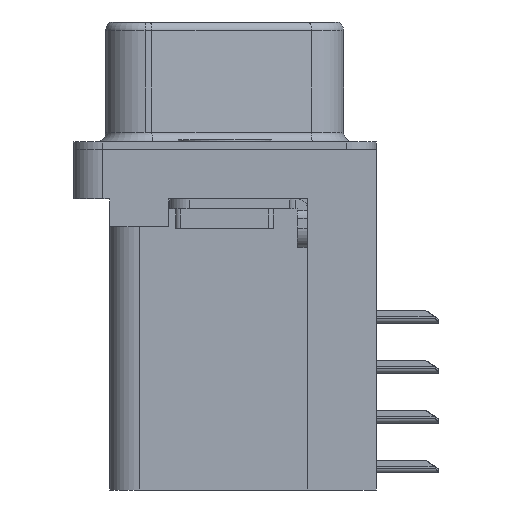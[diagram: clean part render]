
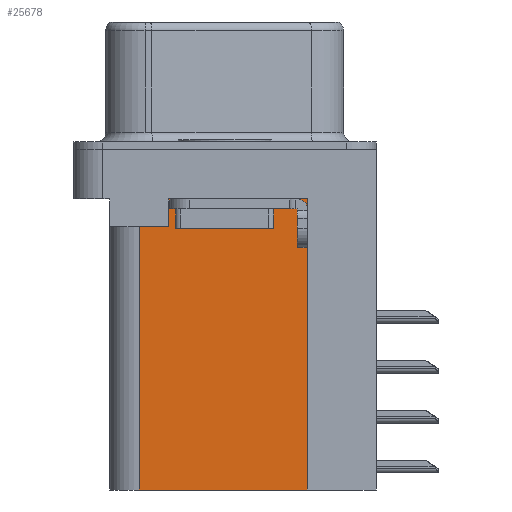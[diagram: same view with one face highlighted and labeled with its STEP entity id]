
A CAD part, left-side view. The second image highlights one B-rep face of the part: STEP entity #25678.
In plain terms, the highlighted planar face has unit normal (-1, 0, 0).
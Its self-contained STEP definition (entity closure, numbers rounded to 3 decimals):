
#505 = EDGE_CURVE ( 'NONE', #12162, #2214, #28429, .T. ) ;
#536 = ORIENTED_EDGE ( 'NONE', *, *, #505, .F. ) ;
#2214 = VERTEX_POINT ( 'NONE', #15525 ) ;
#2223 = ORIENTED_EDGE ( 'NONE', *, *, #35349, .T. ) ;
#3268 = LINE ( 'NONE', #4324, #18031 ) ;
#3417 = CARTESIAN_POINT ( 'NONE',  ( 3.75, 2.85, -3.9 ) ) ;
#3511 = EDGE_CURVE ( 'NONE', #12162, #10727, #16352, .T. ) ;
#3891 = VECTOR ( 'NONE', #4396, 1000. ) ;
#4324 = CARTESIAN_POINT ( 'NONE',  ( 3.75, 4.35, -17.3 ) ) ;
#4396 = DIRECTION ( 'NONE',  ( 0., 1., 0. ) ) ;
#5927 = LINE ( 'NONE', #22564, #13668 ) ;
#7826 = DIRECTION ( 'NONE',  ( 0., 1., 0. ) ) ;
#8161 = VERTEX_POINT ( 'NONE', #13771 ) ;
#8229 = VECTOR ( 'NONE', #20937, 1000. ) ;
#9445 = AXIS2_PLACEMENT_3D ( 'NONE', #10830, #38071, #19734 ) ;
#10727 = VERTEX_POINT ( 'NONE', #12893 ) ;
#10830 = CARTESIAN_POINT ( 'NONE',  ( 3.75, -4.2, -17.3 ) ) ;
#11725 = LINE ( 'NONE', #16073, #3891 ) ;
#12074 = CARTESIAN_POINT ( 'NONE',  ( 3.75, -4.2, -17.3 ) ) ;
#12162 = VERTEX_POINT ( 'NONE', #12074 ) ;
#12893 = CARTESIAN_POINT ( 'NONE',  ( 3.75, -4.2, -2.5 ) ) ;
#13668 = VECTOR ( 'NONE', #7826, 1000. ) ;
#13771 = CARTESIAN_POINT ( 'NONE',  ( 3.75, 2.85, -2.5 ) ) ;
#14056 = EDGE_CURVE ( 'NONE', #23546, #19705, #5927, .T. ) ;
#15314 = ORIENTED_EDGE ( 'NONE', *, *, #3511, .T. ) ;
#15402 = VECTOR ( 'NONE', #32599, 1000. ) ;
#15525 = CARTESIAN_POINT ( 'NONE',  ( 3.75, 4.35, -17.3 ) ) ;
#16073 = CARTESIAN_POINT ( 'NONE',  ( 3.75, -4.2, -2.5 ) ) ;
#16142 = DIRECTION ( 'NONE',  ( 0., 0., 1. ) ) ;
#16352 = LINE ( 'NONE', #33920, #15402 ) ;
#18031 = VECTOR ( 'NONE', #16142, 1000. ) ;
#19467 = EDGE_CURVE ( 'NONE', #10727, #8161, #11725, .T. ) ;
#19604 = PLANE ( 'NONE',  #9445 ) ;
#19705 = VERTEX_POINT ( 'NONE', #20159 ) ;
#19734 = DIRECTION ( 'NONE',  ( 0., 1., 0. ) ) ;
#20159 = CARTESIAN_POINT ( 'NONE',  ( 3.75, 4.35, -3.9 ) ) ;
#20937 = DIRECTION ( 'NONE',  ( 0., 0., -1. ) ) ;
#21543 = ORIENTED_EDGE ( 'NONE', *, *, #19467, .T. ) ;
#22564 = CARTESIAN_POINT ( 'NONE',  ( 3.75, 0., -3.9 ) ) ;
#23546 = VERTEX_POINT ( 'NONE', #3417 ) ;
#23863 = DIRECTION ( 'NONE',  ( 0., 1., 0. ) ) ;
#25678 = ADVANCED_FACE ( 'NONE', ( #29738 ), #19604, .F. ) ;
#27247 = ORIENTED_EDGE ( 'NONE', *, *, #14056, .T. ) ;
#27482 = VECTOR ( 'NONE', #23863, 1000. ) ;
#28429 = LINE ( 'NONE', #29606, #27482 ) ;
#29606 = CARTESIAN_POINT ( 'NONE',  ( 3.75, -4.2, -17.3 ) ) ;
#29738 = FACE_OUTER_BOUND ( 'NONE', #36845, .T. ) ;
#30799 = ORIENTED_EDGE ( 'NONE', *, *, #33049, .F. ) ;
#32108 = LINE ( 'NONE', #35957, #8229 ) ;
#32599 = DIRECTION ( 'NONE',  ( 0., 0., 1. ) ) ;
#33049 = EDGE_CURVE ( 'NONE', #2214, #19705, #3268, .T. ) ;
#33920 = CARTESIAN_POINT ( 'NONE',  ( 3.75, -4.2, -17.3 ) ) ;
#35349 = EDGE_CURVE ( 'NONE', #8161, #23546, #32108, .T. ) ;
#35957 = CARTESIAN_POINT ( 'NONE',  ( 3.75, 2.85, -3.9 ) ) ;
#36845 = EDGE_LOOP ( 'NONE', ( #21543, #2223, #27247, #30799, #536, #15314 ) ) ;
#38071 = DIRECTION ( 'NONE',  ( 1., 0., 0. ) ) ;
